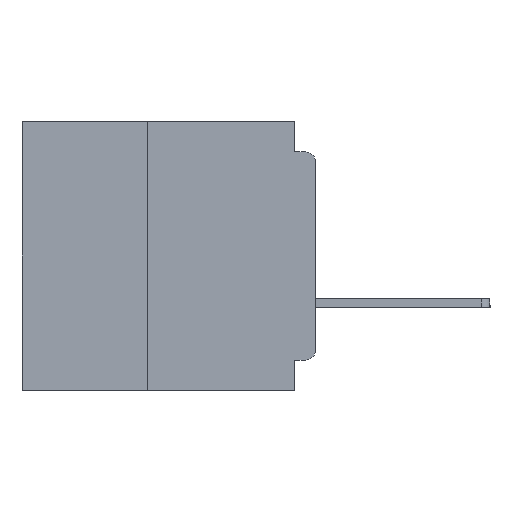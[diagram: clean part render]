
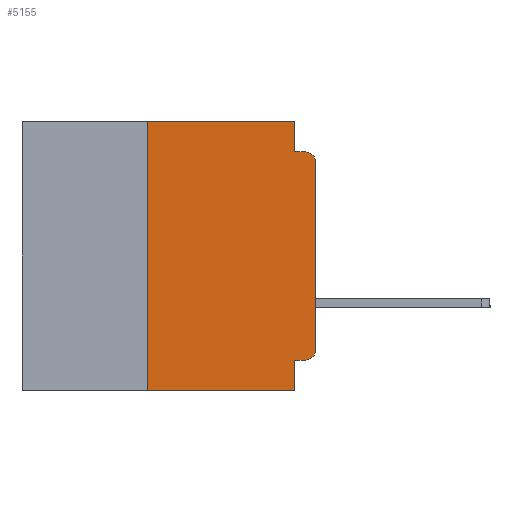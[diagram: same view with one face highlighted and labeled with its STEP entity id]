
A CAD part, left-side view. The second image highlights one B-rep face of the part: STEP entity #5155.
In plain terms, the highlighted planar face has unit normal (-1, 0, 0).
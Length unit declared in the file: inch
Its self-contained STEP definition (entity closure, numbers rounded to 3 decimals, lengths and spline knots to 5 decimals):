
#224 = EDGE_CURVE ( 'NONE', #38522, #7171, #35210, .T. ) ;
#254 = CARTESIAN_POINT ( 'NONE',  ( 0., 0.031, -0.045 ) ) ;
#284 = DIRECTION ( 'NONE',  ( 0., 0., 1. ) ) ;
#297 = EDGE_CURVE ( 'NONE', #22586, #38522, #40228, .T. ) ;
#409 = DIRECTION ( 'NONE',  ( 0., -1., 0. ) ) ;
#632 = DIRECTION ( 'NONE',  ( 0., 0., -1. ) ) ;
#1671 = EDGE_CURVE ( 'NONE', #6076, #15641, #25994, .T. ) ;
#1783 = VECTOR ( 'NONE', #31090, 39.37008 ) ;
#2024 = VERTEX_POINT ( 'NONE', #44540 ) ;
#3294 = VECTOR ( 'NONE', #36821, 39.37008 ) ;
#3452 = LINE ( 'NONE', #34115, #40732 ) ;
#3862 = CARTESIAN_POINT ( 'NONE',  ( 0., 0.031, -0.355 ) ) ;
#5155 = ADVANCED_FACE ( 'NONE', ( #22326 ), #17159, .F. ) ;
#5799 = CARTESIAN_POINT ( 'NONE',  ( 0., 0.031, 0. ) ) ;
#5941 = LINE ( 'NONE', #37996, #43202 ) ;
#6048 = DIRECTION ( 'NONE',  ( 0., 1., 0. ) ) ;
#6076 = VERTEX_POINT ( 'NONE', #11643 ) ;
#7171 = VERTEX_POINT ( 'NONE', #38528 ) ;
#9125 = DIRECTION ( 'NONE',  ( 0., -1., 0. ) ) ;
#9416 = ORIENTED_EDGE ( 'NONE', *, *, #15445, .F. ) ;
#9438 = EDGE_CURVE ( 'NONE', #41515, #25093, #19939, .T. ) ;
#10914 = ORIENTED_EDGE ( 'NONE', *, *, #32148, .T. ) ;
#11404 = VECTOR ( 'NONE', #284, 39.37008 ) ;
#11543 = AXIS2_PLACEMENT_3D ( 'NONE', #42383, #20815, #45966 ) ;
#11643 = CARTESIAN_POINT ( 'NONE',  ( 0., 0.25, -0.4 ) ) ;
#12433 = DIRECTION ( 'NONE',  ( 0., 0., -1. ) ) ;
#13410 = CIRCLE ( 'NONE', #37503, 0.015 ) ;
#14052 = LINE ( 'NONE', #33209, #3294 ) ;
#14232 = LINE ( 'NONE', #24102, #40744 ) ;
#15445 = EDGE_CURVE ( 'NONE', #28311, #41472, #14232, .T. ) ;
#15641 = VERTEX_POINT ( 'NONE', #45221 ) ;
#15749 = ORIENTED_EDGE ( 'NONE', *, *, #9438, .F. ) ;
#16308 = VECTOR ( 'NONE', #409, 39.37008 ) ;
#17142 = CARTESIAN_POINT ( 'NONE',  ( 0., 0.015, -0.34 ) ) ;
#17159 = PLANE ( 'NONE',  #11543 ) ;
#18255 = ORIENTED_EDGE ( 'NONE', *, *, #224, .T. ) ;
#19144 = EDGE_CURVE ( 'NONE', #15641, #41515, #5941, .T. ) ;
#19939 = LINE ( 'NONE', #5799, #1783 ) ;
#20602 = ORIENTED_EDGE ( 'NONE', *, *, #43965, .T. ) ;
#20793 = DIRECTION ( 'NONE',  ( 0., 0., -1. ) ) ;
#20815 = DIRECTION ( 'NONE',  ( 1., 0., 0. ) ) ;
#21062 = ORIENTED_EDGE ( 'NONE', *, *, #1671, .F. ) ;
#21249 = CARTESIAN_POINT ( 'NONE',  ( 0., 0., -0.34 ) ) ;
#22326 = FACE_OUTER_BOUND ( 'NONE', #24223, .T. ) ;
#22586 = VERTEX_POINT ( 'NONE', #21249 ) ;
#24102 = CARTESIAN_POINT ( 'NONE',  ( 0., 0., -0.355 ) ) ;
#24223 = EDGE_LOOP ( 'NONE', ( #42451, #18255, #46195, #15749, #35683, #21062, #10914, #28937, #9416, #20602 ) ) ;
#24657 = DIRECTION ( 'NONE',  ( -1., 0., 0. ) ) ;
#25093 = VERTEX_POINT ( 'NONE', #254 ) ;
#25994 = LINE ( 'NONE', #39142, #33346 ) ;
#27604 = CARTESIAN_POINT ( 'NONE',  ( 0., 0., -0.06 ) ) ;
#28213 = LINE ( 'NONE', #43485, #16308 ) ;
#28293 = EDGE_CURVE ( 'NONE', #41472, #2024, #3452, .T. ) ;
#28311 = VERTEX_POINT ( 'NONE', #45082 ) ;
#28937 = ORIENTED_EDGE ( 'NONE', *, *, #28293, .F. ) ;
#31090 = DIRECTION ( 'NONE',  ( 0., 0., -1. ) ) ;
#32148 = EDGE_CURVE ( 'NONE', #6076, #2024, #14052, .T. ) ;
#32837 = CARTESIAN_POINT ( 'NONE',  ( 0., 0., 0. ) ) ;
#33209 = CARTESIAN_POINT ( 'NONE',  ( 0., 0.437, -0.4 ) ) ;
#33346 = VECTOR ( 'NONE', #36463, 39.37008 ) ;
#34115 = CARTESIAN_POINT ( 'NONE',  ( 0., 0.031, -0.4 ) ) ;
#35210 = CIRCLE ( 'NONE', #39227, 0.015 ) ;
#35683 = ORIENTED_EDGE ( 'NONE', *, *, #19144, .F. ) ;
#36463 = DIRECTION ( 'NONE',  ( 0., 0., 1. ) ) ;
#36821 = DIRECTION ( 'NONE',  ( 0., -1., 0. ) ) ;
#37503 = AXIS2_PLACEMENT_3D ( 'NONE', #17142, #42370, #20793 ) ;
#37996 = CARTESIAN_POINT ( 'NONE',  ( 0., 0.437, 0. ) ) ;
#38522 = VERTEX_POINT ( 'NONE', #27604 ) ;
#38528 = CARTESIAN_POINT ( 'NONE',  ( 0., 0.015, -0.045 ) ) ;
#39142 = CARTESIAN_POINT ( 'NONE',  ( 0., 0.25, -0.4 ) ) ;
#39227 = AXIS2_PLACEMENT_3D ( 'NONE', #39907, #24657, #632 ) ;
#39907 = CARTESIAN_POINT ( 'NONE',  ( 0., 0.015, -0.06 ) ) ;
#40228 = LINE ( 'NONE', #32837, #11404 ) ;
#40732 = VECTOR ( 'NONE', #12433, 39.37008 ) ;
#40744 = VECTOR ( 'NONE', #6048, 39.37008 ) ;
#41472 = VERTEX_POINT ( 'NONE', #3862 ) ;
#41498 = EDGE_CURVE ( 'NONE', #25093, #7171, #28213, .T. ) ;
#41515 = VERTEX_POINT ( 'NONE', #43785 ) ;
#42370 = DIRECTION ( 'NONE',  ( -1., 0., 0. ) ) ;
#42383 = CARTESIAN_POINT ( 'NONE',  ( 0., 0.437, 0. ) ) ;
#42451 = ORIENTED_EDGE ( 'NONE', *, *, #297, .T. ) ;
#43202 = VECTOR ( 'NONE', #9125, 39.37008 ) ;
#43485 = CARTESIAN_POINT ( 'NONE',  ( 0., 0., -0.045 ) ) ;
#43785 = CARTESIAN_POINT ( 'NONE',  ( 0., 0.031, 0. ) ) ;
#43965 = EDGE_CURVE ( 'NONE', #28311, #22586, #13410, .T. ) ;
#44540 = CARTESIAN_POINT ( 'NONE',  ( 0., 0.031, -0.4 ) ) ;
#45082 = CARTESIAN_POINT ( 'NONE',  ( 0., 0.015, -0.355 ) ) ;
#45221 = CARTESIAN_POINT ( 'NONE',  ( 0., 0.25, 0. ) ) ;
#45966 = DIRECTION ( 'NONE',  ( 0., 0., -1. ) ) ;
#46195 = ORIENTED_EDGE ( 'NONE', *, *, #41498, .F. ) ;
